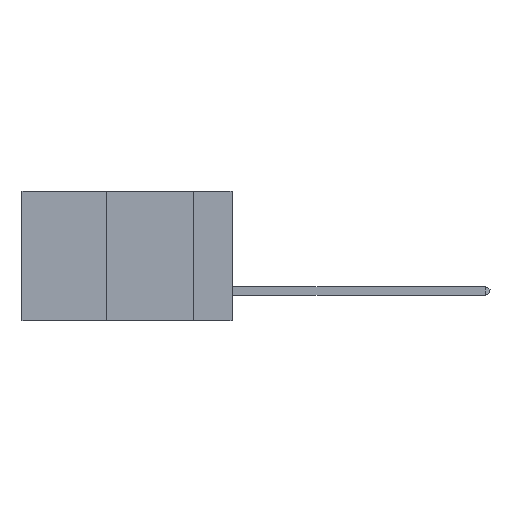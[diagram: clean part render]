
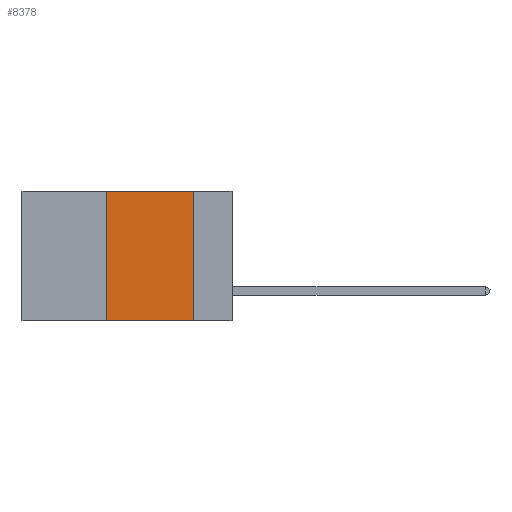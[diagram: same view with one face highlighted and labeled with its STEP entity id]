
A CAD part, left-side view. The second image highlights one B-rep face of the part: STEP entity #8378.
In plain terms, the highlighted planar face has unit normal (-1, 0, 0).
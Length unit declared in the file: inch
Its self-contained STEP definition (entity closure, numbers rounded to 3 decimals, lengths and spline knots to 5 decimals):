
#485 = CARTESIAN_POINT ( 'NONE',  ( 0., 0.36, 0. ) ) ;
#585 = FACE_OUTER_BOUND ( 'NONE', #11915, .T. ) ;
#662 = PLANE ( 'NONE',  #4765 ) ;
#1177 = DIRECTION ( 'NONE',  ( 0., 0., -1. ) ) ;
#1667 = DIRECTION ( 'NONE',  ( 1., 0., 0. ) ) ;
#1696 = LINE ( 'NONE', #2164, #3134 ) ;
#2164 = CARTESIAN_POINT ( 'NONE',  ( 0., 0.11, 0. ) ) ;
#3134 = VECTOR ( 'NONE', #1177, 39.37008 ) ;
#3309 = VECTOR ( 'NONE', #7159, 39.37008 ) ;
#3693 = EDGE_CURVE ( 'NONE', #4022, #11043, #4175, .T. ) ;
#4022 = VERTEX_POINT ( 'NONE', #485 ) ;
#4175 = LINE ( 'NONE', #9729, #3309 ) ;
#4299 = EDGE_CURVE ( 'NONE', #6696, #11925, #11395, .T. ) ;
#4327 = DIRECTION ( 'NONE',  ( 0., -1., 0. ) ) ;
#4435 = VECTOR ( 'NONE', #4327, 39.37008 ) ;
#4765 = AXIS2_PLACEMENT_3D ( 'NONE', #8905, #1667, #9645 ) ;
#5176 = EDGE_CURVE ( 'NONE', #11043, #11925, #1696, .T. ) ;
#5336 = ORIENTED_EDGE ( 'NONE', *, *, #3693, .F. ) ;
#5971 = CARTESIAN_POINT ( 'NONE',  ( 0., 0.11, 0. ) ) ;
#6088 = CARTESIAN_POINT ( 'NONE',  ( 0., 0.36, -0.37 ) ) ;
#6667 = CARTESIAN_POINT ( 'NONE',  ( 0., 0.36, 0. ) ) ;
#6696 = VERTEX_POINT ( 'NONE', #6088 ) ;
#7159 = DIRECTION ( 'NONE',  ( 0., -1., 0. ) ) ;
#7263 = ORIENTED_EDGE ( 'NONE', *, *, #7821, .F. ) ;
#7389 = CARTESIAN_POINT ( 'NONE',  ( 0., 0.11, -0.37 ) ) ;
#7821 = EDGE_CURVE ( 'NONE', #6696, #4022, #7852, .T. ) ;
#7852 = LINE ( 'NONE', #6667, #10902 ) ;
#8378 = ADVANCED_FACE ( 'NONE', ( #585 ), #662, .F. ) ;
#8905 = CARTESIAN_POINT ( 'NONE',  ( 0., 0.6, 0. ) ) ;
#9229 = ORIENTED_EDGE ( 'NONE', *, *, #4299, .T. ) ;
#9645 = DIRECTION ( 'NONE',  ( 0., 0., -1. ) ) ;
#9729 = CARTESIAN_POINT ( 'NONE',  ( 0., 0.6, 0. ) ) ;
#9813 = ORIENTED_EDGE ( 'NONE', *, *, #5176, .F. ) ;
#10381 = DIRECTION ( 'NONE',  ( 0., 0., 1. ) ) ;
#10776 = CARTESIAN_POINT ( 'NONE',  ( 0., 0.6, -0.37 ) ) ;
#10902 = VECTOR ( 'NONE', #10381, 39.37008 ) ;
#11043 = VERTEX_POINT ( 'NONE', #5971 ) ;
#11395 = LINE ( 'NONE', #10776, #4435 ) ;
#11915 = EDGE_LOOP ( 'NONE', ( #9813, #5336, #7263, #9229 ) ) ;
#11925 = VERTEX_POINT ( 'NONE', #7389 ) ;
